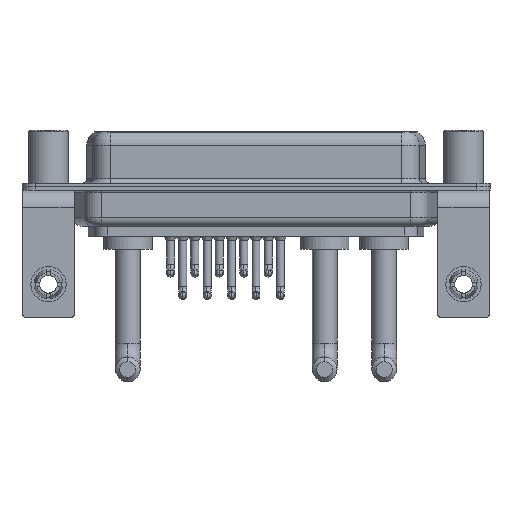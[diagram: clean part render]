
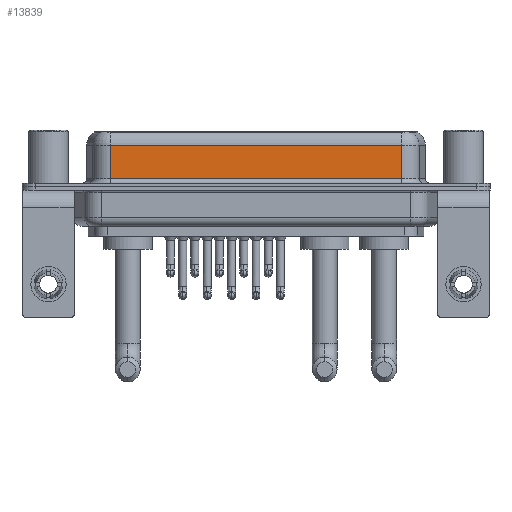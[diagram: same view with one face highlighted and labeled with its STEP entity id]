
A CAD part, front view. The second image highlights one B-rep face of the part: STEP entity #13839.
In plain terms, the highlighted planar face has unit normal (0, -1, 0).
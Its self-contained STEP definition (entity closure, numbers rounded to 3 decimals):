
#677 = EDGE_CURVE ( 'NONE', #16786, #19519, #793, .T. ) ;
#792 = CARTESIAN_POINT ( 'NONE',  ( 40.037, -3.95, 6.4 ) ) ;
#793 = LINE ( 'NONE', #13356, #21325 ) ;
#1356 = CARTESIAN_POINT ( 'NONE',  ( 7.013, -3.95, 0.9 ) ) ;
#2037 = EDGE_CURVE ( 'NONE', #19519, #11350, #12055, .T. ) ;
#3498 = VERTEX_POINT ( 'NONE', #17996 ) ;
#3667 = VECTOR ( 'NONE', #22098, 1000. ) ;
#3852 = AXIS2_PLACEMENT_3D ( 'NONE', #792, #11591, #11815 ) ;
#5046 = DIRECTION ( 'NONE',  ( 1., 0., 0. ) ) ;
#6408 = PLANE ( 'NONE',  #3852 ) ;
#7717 = CARTESIAN_POINT ( 'NONE',  ( 7.013, -3.95, 4.65 ) ) ;
#10291 = DIRECTION ( 'NONE',  ( 0., 0., -1. ) ) ;
#10498 = VECTOR ( 'NONE', #10291, 1000. ) ;
#10949 = CARTESIAN_POINT ( 'NONE',  ( 40.037, -3.95, 6.4 ) ) ;
#11058 = ORIENTED_EDGE ( 'NONE', *, *, #677, .T. ) ;
#11350 = VERTEX_POINT ( 'NONE', #1356 ) ;
#11591 = DIRECTION ( 'NONE',  ( 0., 1., 0. ) ) ;
#11593 = DIRECTION ( 'NONE',  ( -1., 0., 0. ) ) ;
#11815 = DIRECTION ( 'NONE',  ( 0., 0., 1. ) ) ;
#12055 = LINE ( 'NONE', #19205, #10498 ) ;
#12684 = EDGE_CURVE ( 'NONE', #16786, #3498, #14941, .T. ) ;
#13079 = EDGE_LOOP ( 'NONE', ( #18340, #11058, #22770, #19352 ) ) ;
#13134 = EDGE_CURVE ( 'NONE', #11350, #3498, #17492, .T. ) ;
#13356 = CARTESIAN_POINT ( 'NONE',  ( 40.037, -3.95, 4.65 ) ) ;
#13839 = ADVANCED_FACE ( 'NONE', ( #16988 ), #6408, .F. ) ;
#14941 = LINE ( 'NONE', #10949, #3667 ) ;
#16786 = VERTEX_POINT ( 'NONE', #22305 ) ;
#16988 = FACE_OUTER_BOUND ( 'NONE', #13079, .T. ) ;
#17492 = LINE ( 'NONE', #23112, #19682 ) ;
#17996 = CARTESIAN_POINT ( 'NONE',  ( 40.037, -3.95, 0.9 ) ) ;
#18340 = ORIENTED_EDGE ( 'NONE', *, *, #12684, .F. ) ;
#19205 = CARTESIAN_POINT ( 'NONE',  ( 7.013, -3.95, 6.4 ) ) ;
#19352 = ORIENTED_EDGE ( 'NONE', *, *, #13134, .T. ) ;
#19519 = VERTEX_POINT ( 'NONE', #7717 ) ;
#19682 = VECTOR ( 'NONE', #5046, 1000. ) ;
#21325 = VECTOR ( 'NONE', #11593, 1000. ) ;
#22098 = DIRECTION ( 'NONE',  ( 0., 0., -1. ) ) ;
#22305 = CARTESIAN_POINT ( 'NONE',  ( 40.037, -3.95, 4.65 ) ) ;
#22770 = ORIENTED_EDGE ( 'NONE', *, *, #2037, .T. ) ;
#23112 = CARTESIAN_POINT ( 'NONE',  ( 40.037, -3.95, 0.9 ) ) ;
